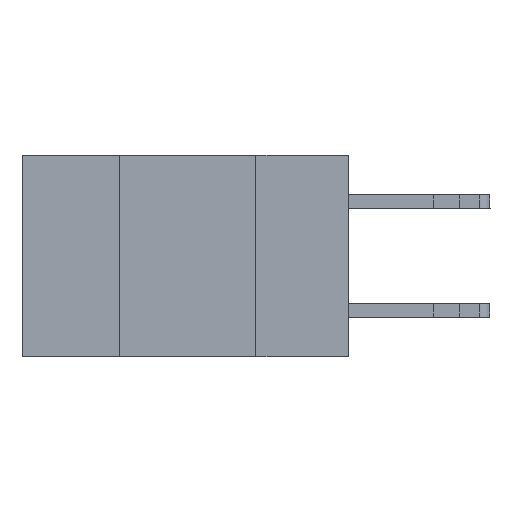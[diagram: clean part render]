
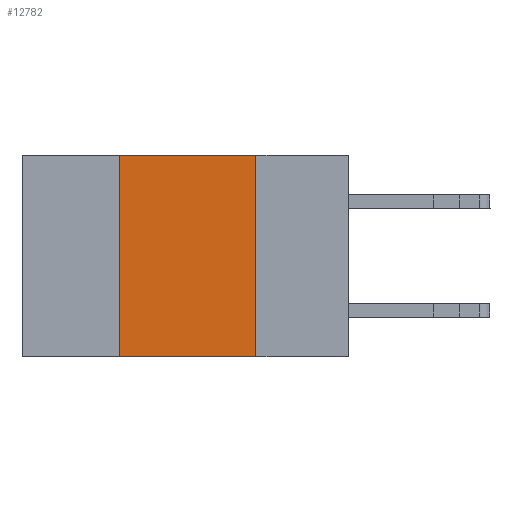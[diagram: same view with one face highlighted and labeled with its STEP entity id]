
A CAD part, left-side view. The second image highlights one B-rep face of the part: STEP entity #12782.
In plain terms, the highlighted planar face has unit normal (-1, 0, 0).
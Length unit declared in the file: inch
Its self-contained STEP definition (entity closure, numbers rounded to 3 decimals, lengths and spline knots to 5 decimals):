
#387 = VECTOR ( 'NONE', #21780, 39.37008 ) ;
#691 = EDGE_CURVE ( 'NONE', #14135, #18541, #15763, .T. ) ;
#1102 = CARTESIAN_POINT ( 'NONE',  ( 0., 0.42, -0.37 ) ) ;
#2483 = EDGE_CURVE ( 'NONE', #12248, #14135, #3459, .T. ) ;
#3017 = DIRECTION ( 'NONE',  ( 1., 0., 0. ) ) ;
#3218 = ORIENTED_EDGE ( 'NONE', *, *, #2483, .F. ) ;
#3459 = LINE ( 'NONE', #10426, #7914 ) ;
#3817 = ORIENTED_EDGE ( 'NONE', *, *, #18284, .T. ) ;
#4349 = LINE ( 'NONE', #17341, #22390 ) ;
#4952 = VERTEX_POINT ( 'NONE', #22563 ) ;
#6091 = LINE ( 'NONE', #12408, #387 ) ;
#6806 = AXIS2_PLACEMENT_3D ( 'NONE', #8642, #3017, #16082 ) ;
#7914 = VECTOR ( 'NONE', #21561, 39.37008 ) ;
#8642 = CARTESIAN_POINT ( 'NONE',  ( 0., 0.6, 0. ) ) ;
#9026 = EDGE_LOOP ( 'NONE', ( #24178, #16361, #3218, #3817 ) ) ;
#10426 = CARTESIAN_POINT ( 'NONE',  ( 0., 0.42, -0.37 ) ) ;
#11195 = CARTESIAN_POINT ( 'NONE',  ( 0., 0.17, 0. ) ) ;
#12010 = EDGE_CURVE ( 'NONE', #18541, #4952, #4349, .T. ) ;
#12248 = VERTEX_POINT ( 'NONE', #1102 ) ;
#12303 = PLANE ( 'NONE',  #6806 ) ;
#12408 = CARTESIAN_POINT ( 'NONE',  ( 0., 0.6, -0.37 ) ) ;
#12782 = ADVANCED_FACE ( 'NONE', ( #20348 ), #12303, .F. ) ;
#13638 = DIRECTION ( 'NONE',  ( 0., 0., -1. ) ) ;
#14050 = CARTESIAN_POINT ( 'NONE',  ( 0., 0.42, 0. ) ) ;
#14135 = VERTEX_POINT ( 'NONE', #14050 ) ;
#15763 = LINE ( 'NONE', #17759, #21284 ) ;
#16082 = DIRECTION ( 'NONE',  ( 0., 0., -1. ) ) ;
#16361 = ORIENTED_EDGE ( 'NONE', *, *, #691, .F. ) ;
#17341 = CARTESIAN_POINT ( 'NONE',  ( 0., 0.17, -0.37 ) ) ;
#17753 = DIRECTION ( 'NONE',  ( 0., -1., 0. ) ) ;
#17759 = CARTESIAN_POINT ( 'NONE',  ( 0., 0.6, 0. ) ) ;
#18284 = EDGE_CURVE ( 'NONE', #12248, #4952, #6091, .T. ) ;
#18541 = VERTEX_POINT ( 'NONE', #11195 ) ;
#20348 = FACE_OUTER_BOUND ( 'NONE', #9026, .T. ) ;
#21284 = VECTOR ( 'NONE', #17753, 39.37008 ) ;
#21561 = DIRECTION ( 'NONE',  ( 0., 0., 1. ) ) ;
#21780 = DIRECTION ( 'NONE',  ( 0., -1., 0. ) ) ;
#22390 = VECTOR ( 'NONE', #13638, 39.37008 ) ;
#22563 = CARTESIAN_POINT ( 'NONE',  ( 0., 0.17, -0.37 ) ) ;
#24178 = ORIENTED_EDGE ( 'NONE', *, *, #12010, .F. ) ;
